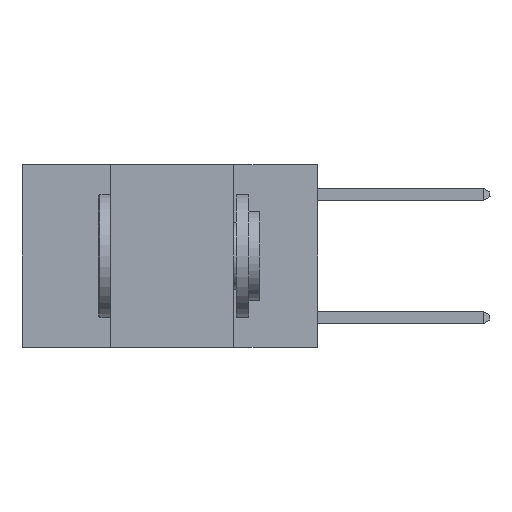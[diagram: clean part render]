
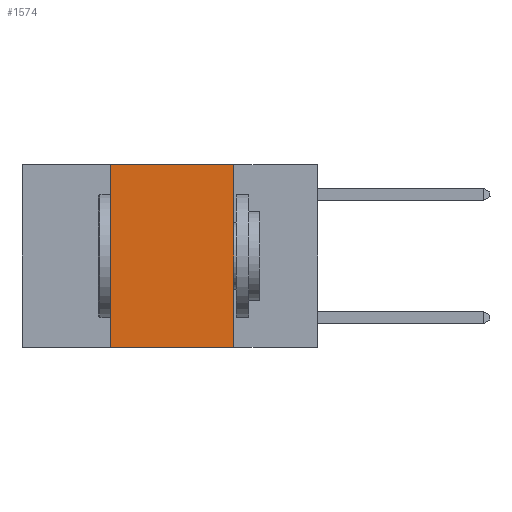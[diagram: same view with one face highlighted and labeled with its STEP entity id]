
A CAD part, left-side view. The second image highlights one B-rep face of the part: STEP entity #1574.
In plain terms, the highlighted planar face has unit normal (-1, 0, 0).
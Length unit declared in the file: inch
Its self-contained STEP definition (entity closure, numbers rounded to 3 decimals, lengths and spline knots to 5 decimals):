
#127 = DIRECTION ( 'NONE',  ( 0., 0., -1. ) ) ;
#242 = LINE ( 'NONE', #2794, #8159 ) ;
#485 = VECTOR ( 'NONE', #5369, 39.37008 ) ;
#516 = DIRECTION ( 'NONE',  ( 0., 0., -1. ) ) ;
#604 = CARTESIAN_POINT ( 'NONE',  ( 0., 0.6, 0. ) ) ;
#1354 = PLANE ( 'NONE',  #2304 ) ;
#1574 = ADVANCED_FACE ( 'NONE', ( #4605 ), #1354, .F. ) ;
#2169 = LINE ( 'NONE', #7983, #485 ) ;
#2304 = AXIS2_PLACEMENT_3D ( 'NONE', #5501, #2912, #516 ) ;
#2616 = VECTOR ( 'NONE', #5761, 39.37008 ) ;
#2794 = CARTESIAN_POINT ( 'NONE',  ( 0., 0.17, 0. ) ) ;
#2912 = DIRECTION ( 'NONE',  ( 1., 0., 0. ) ) ;
#3470 = VECTOR ( 'NONE', #5732, 39.37008 ) ;
#4242 = ORIENTED_EDGE ( 'NONE', *, *, #8456, .F. ) ;
#4317 = ORIENTED_EDGE ( 'NONE', *, *, #8220, .F. ) ;
#4416 = CARTESIAN_POINT ( 'NONE',  ( 0., 0.17, -0.37 ) ) ;
#4489 = CARTESIAN_POINT ( 'NONE',  ( 0., 0.42, 0. ) ) ;
#4605 = FACE_OUTER_BOUND ( 'NONE', #9681, .T. ) ;
#5369 = DIRECTION ( 'NONE',  ( 0., -1., 0. ) ) ;
#5501 = CARTESIAN_POINT ( 'NONE',  ( 0., 0.6, 0. ) ) ;
#5672 = EDGE_CURVE ( 'NONE', #7604, #7722, #6577, .T. ) ;
#5732 = DIRECTION ( 'NONE',  ( 0., 0., 1. ) ) ;
#5761 = DIRECTION ( 'NONE',  ( 0., -1., 0. ) ) ;
#6577 = LINE ( 'NONE', #10908, #3470 ) ;
#7158 = CARTESIAN_POINT ( 'NONE',  ( 0., 0.17, 0. ) ) ;
#7604 = VERTEX_POINT ( 'NONE', #10455 ) ;
#7722 = VERTEX_POINT ( 'NONE', #4489 ) ;
#7983 = CARTESIAN_POINT ( 'NONE',  ( 0., 0.6, -0.37 ) ) ;
#8105 = ORIENTED_EDGE ( 'NONE', *, *, #5672, .F. ) ;
#8159 = VECTOR ( 'NONE', #127, 39.37008 ) ;
#8220 = EDGE_CURVE ( 'NONE', #8291, #9131, #242, .T. ) ;
#8291 = VERTEX_POINT ( 'NONE', #7158 ) ;
#8301 = ORIENTED_EDGE ( 'NONE', *, *, #8736, .T. ) ;
#8456 = EDGE_CURVE ( 'NONE', #7722, #8291, #9203, .T. ) ;
#8736 = EDGE_CURVE ( 'NONE', #7604, #9131, #2169, .T. ) ;
#9131 = VERTEX_POINT ( 'NONE', #4416 ) ;
#9203 = LINE ( 'NONE', #604, #2616 ) ;
#9681 = EDGE_LOOP ( 'NONE', ( #4317, #4242, #8105, #8301 ) ) ;
#10455 = CARTESIAN_POINT ( 'NONE',  ( 0., 0.42, -0.37 ) ) ;
#10908 = CARTESIAN_POINT ( 'NONE',  ( 0., 0.42, 0. ) ) ;
